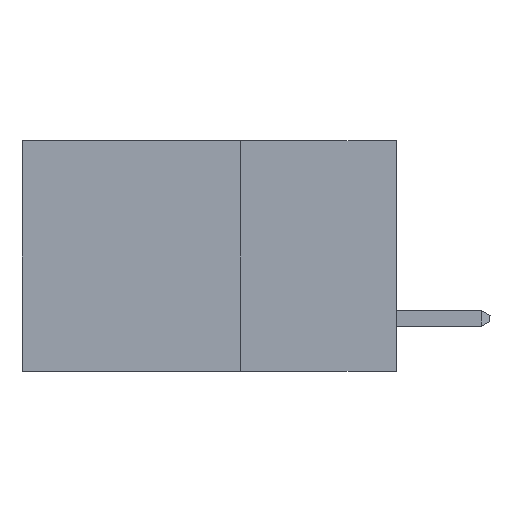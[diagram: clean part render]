
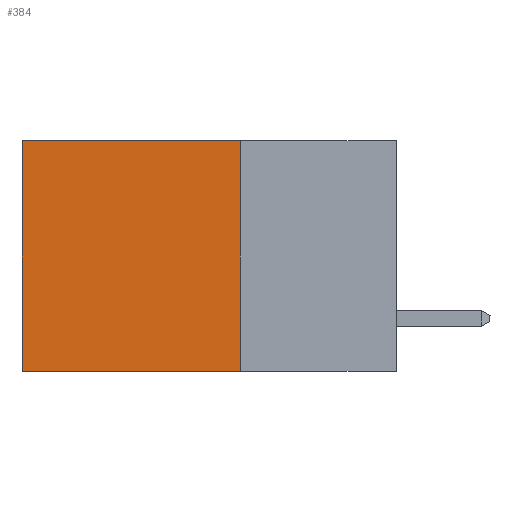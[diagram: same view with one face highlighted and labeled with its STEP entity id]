
A CAD part, left-side view. The second image highlights one B-rep face of the part: STEP entity #384.
In plain terms, the highlighted planar face has unit normal (-1, 0, 0).
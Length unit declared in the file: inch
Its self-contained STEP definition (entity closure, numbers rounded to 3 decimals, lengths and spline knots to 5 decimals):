
#384 = ADVANCED_FACE ( 'NONE', ( #3355 ), #11047, .F. ) ;
#1619 = VERTEX_POINT ( 'NONE', #11098 ) ;
#1624 = VECTOR ( 'NONE', #5327, 39.37008 ) ;
#2185 = EDGE_LOOP ( 'NONE', ( #9132, #8812, #15678, #4209 ) ) ;
#2691 = VECTOR ( 'NONE', #14168, 39.37008 ) ;
#3289 = LINE ( 'NONE', #9999, #3670 ) ;
#3355 = FACE_OUTER_BOUND ( 'NONE', #2185, .T. ) ;
#3670 = VECTOR ( 'NONE', #15189, 39.37008 ) ;
#4105 = CARTESIAN_POINT ( 'NONE',  ( 0.2615, 0.25, 0. ) ) ;
#4209 = ORIENTED_EDGE ( 'NONE', *, *, #13123, .T. ) ;
#5327 = DIRECTION ( 'NONE',  ( 0., 1., 0. ) ) ;
#5359 = VERTEX_POINT ( 'NONE', #6764 ) ;
#5467 = LINE ( 'NONE', #4105, #1624 ) ;
#6092 = CARTESIAN_POINT ( 'NONE',  ( 0.2615, 0.6, -0.37 ) ) ;
#6764 = CARTESIAN_POINT ( 'NONE',  ( 0.2615, 0.25, -0.37 ) ) ;
#7294 = AXIS2_PLACEMENT_3D ( 'NONE', #10795, #10736, #10608 ) ;
#8812 = ORIENTED_EDGE ( 'NONE', *, *, #12402, .F. ) ;
#9132 = ORIENTED_EDGE ( 'NONE', *, *, #15374, .T. ) ;
#9550 = EDGE_CURVE ( 'NONE', #11046, #5359, #3289, .T. ) ;
#9784 = LINE ( 'NONE', #6092, #16248 ) ;
#9999 = CARTESIAN_POINT ( 'NONE',  ( 0.2615, 0.25, -0.37 ) ) ;
#10214 = CARTESIAN_POINT ( 'NONE',  ( 0.2615, 0.25, -0.37 ) ) ;
#10608 = DIRECTION ( 'NONE',  ( 0., 0., -1. ) ) ;
#10736 = DIRECTION ( 'NONE',  ( 1., 0., 0. ) ) ;
#10795 = CARTESIAN_POINT ( 'NONE',  ( 0.2615, 0.25, -0.37 ) ) ;
#11046 = VERTEX_POINT ( 'NONE', #14546 ) ;
#11047 = PLANE ( 'NONE',  #7294 ) ;
#11098 = CARTESIAN_POINT ( 'NONE',  ( 0.2615, 0.6, 0. ) ) ;
#11176 = VERTEX_POINT ( 'NONE', #15965 ) ;
#12402 = EDGE_CURVE ( 'NONE', #5359, #11176, #12598, .T. ) ;
#12560 = DIRECTION ( 'NONE',  ( 0., 0., -1. ) ) ;
#12598 = LINE ( 'NONE', #10214, #2691 ) ;
#13123 = EDGE_CURVE ( 'NONE', #11046, #1619, #5467, .T. ) ;
#14168 = DIRECTION ( 'NONE',  ( 0., 1., 0. ) ) ;
#14546 = CARTESIAN_POINT ( 'NONE',  ( 0.2615, 0.25, 0. ) ) ;
#15189 = DIRECTION ( 'NONE',  ( 0., 0., -1. ) ) ;
#15374 = EDGE_CURVE ( 'NONE', #1619, #11176, #9784, .T. ) ;
#15678 = ORIENTED_EDGE ( 'NONE', *, *, #9550, .F. ) ;
#15965 = CARTESIAN_POINT ( 'NONE',  ( 0.2615, 0.6, -0.37 ) ) ;
#16248 = VECTOR ( 'NONE', #12560, 39.37008 ) ;
